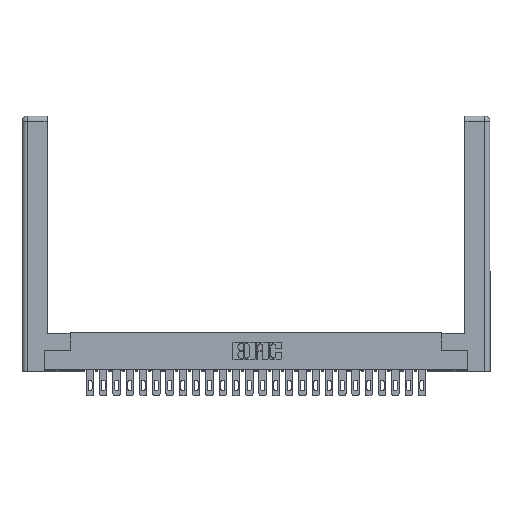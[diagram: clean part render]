
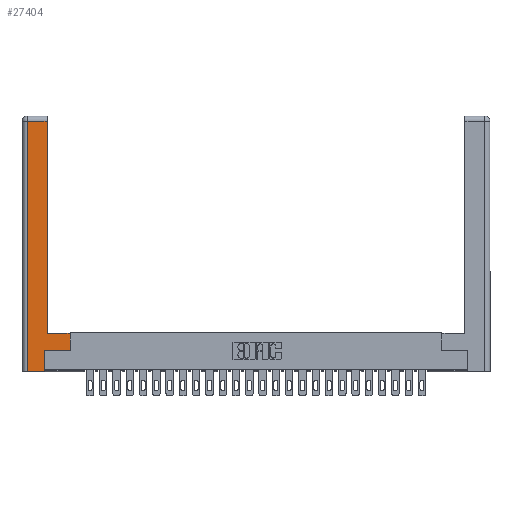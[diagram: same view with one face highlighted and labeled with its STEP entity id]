
A CAD part, top view. The second image highlights one B-rep face of the part: STEP entity #27404.
In plain terms, the highlighted planar face has unit normal (0, 0, 1).
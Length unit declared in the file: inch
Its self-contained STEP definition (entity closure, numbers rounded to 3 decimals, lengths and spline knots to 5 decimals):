
#1443 = ORIENTED_EDGE ( 'NONE', *, *, #8152, .T. ) ;
#1569 = VECTOR ( 'NONE', #4628, 39.37008 ) ;
#1930 = CARTESIAN_POINT ( 'NONE',  ( 0.565, 0.245, 0. ) ) ;
#2510 = VERTEX_POINT ( 'NONE', #10529 ) ;
#3522 = EDGE_CURVE ( 'NONE', #22844, #14500, #9062, .T. ) ;
#3956 = VERTEX_POINT ( 'NONE', #15222 ) ;
#4116 = CARTESIAN_POINT ( 'NONE',  ( 0.265, 0.245, 0. ) ) ;
#4407 = ORIENTED_EDGE ( 'NONE', *, *, #3522, .T. ) ;
#4551 = DIRECTION ( 'NONE',  ( -1., 0., 0. ) ) ;
#4628 = DIRECTION ( 'NONE',  ( -1., 0., 0. ) ) ;
#5605 = EDGE_CURVE ( 'NONE', #5636, #3956, #26532, .T. ) ;
#5636 = VERTEX_POINT ( 'NONE', #1930 ) ;
#5921 = DIRECTION ( 'NONE',  ( 0., -1., 0. ) ) ;
#6219 = DIRECTION ( 'NONE',  ( -1., 0., 0. ) ) ;
#6247 = ORIENTED_EDGE ( 'NONE', *, *, #16109, .T. ) ;
#6635 = CARTESIAN_POINT ( 'NONE',  ( 0.265, 0., 0. ) ) ;
#6903 = AXIS2_PLACEMENT_3D ( 'NONE', #17672, #26797, #4551 ) ;
#7420 = LINE ( 'NONE', #27299, #1569 ) ;
#7659 = ORIENTED_EDGE ( 'NONE', *, *, #13630, .T. ) ;
#7893 = DIRECTION ( 'NONE',  ( 1., 0., 0. ) ) ;
#8052 = VERTEX_POINT ( 'NONE', #11225 ) ;
#8152 = EDGE_CURVE ( 'NONE', #3956, #22844, #7420, .T. ) ;
#8235 = LINE ( 'NONE', #4116, #26697 ) ;
#8256 = EDGE_LOOP ( 'NONE', ( #4407, #15920, #23456, #6247, #7659, #26648, #13505, #1443 ) ) ;
#8911 = DIRECTION ( 'NONE',  ( 0., 1., 0. ) ) ;
#9062 = LINE ( 'NONE', #11106, #13403 ) ;
#10479 = VECTOR ( 'NONE', #7893, 39.37008 ) ;
#10529 = CARTESIAN_POINT ( 'NONE',  ( 0.0615, 0., 0. ) ) ;
#10731 = PLANE ( 'NONE',  #6903 ) ;
#10889 = VECTOR ( 'NONE', #5921, 39.37008 ) ;
#11106 = CARTESIAN_POINT ( 'NONE',  ( 0.295, 3., 0. ) ) ;
#11225 = CARTESIAN_POINT ( 'NONE',  ( 0.0615, 2.94, 0. ) ) ;
#12247 = CARTESIAN_POINT ( 'NONE',  ( 0.295, 0.45, 0. ) ) ;
#12277 = CARTESIAN_POINT ( 'NONE',  ( 0.565, 0.245, 0. ) ) ;
#12647 = CARTESIAN_POINT ( 'NONE',  ( 0.0615, 0., 0. ) ) ;
#12722 = LINE ( 'NONE', #12277, #10479 ) ;
#13403 = VECTOR ( 'NONE', #8911, 39.37008 ) ;
#13505 = ORIENTED_EDGE ( 'NONE', *, *, #5605, .T. ) ;
#13630 = EDGE_CURVE ( 'NONE', #23438, #15552, #8235, .T. ) ;
#14363 = CARTESIAN_POINT ( 'NONE',  ( 0.265, 0.245, 0. ) ) ;
#14500 = VERTEX_POINT ( 'NONE', #28344 ) ;
#15222 = CARTESIAN_POINT ( 'NONE',  ( 0.565, 0.45, 0. ) ) ;
#15308 = FACE_OUTER_BOUND ( 'NONE', #8256, .T. ) ;
#15552 = VERTEX_POINT ( 'NONE', #14363 ) ;
#15601 = DIRECTION ( 'NONE',  ( 1., 0., 0. ) ) ;
#15920 = ORIENTED_EDGE ( 'NONE', *, *, #17751, .T. ) ;
#15979 = VECTOR ( 'NONE', #6219, 39.37008 ) ;
#16109 = EDGE_CURVE ( 'NONE', #2510, #23438, #20025, .T. ) ;
#16445 = CARTESIAN_POINT ( 'NONE',  ( 0.265, 0., 0. ) ) ;
#17672 = CARTESIAN_POINT ( 'NONE',  ( 0., 0., 0. ) ) ;
#17751 = EDGE_CURVE ( 'NONE', #14500, #8052, #28140, .T. ) ;
#20025 = LINE ( 'NONE', #6635, #23934 ) ;
#20279 = EDGE_CURVE ( 'NONE', #8052, #2510, #26665, .T. ) ;
#21168 = EDGE_CURVE ( 'NONE', #15552, #5636, #12722, .T. ) ;
#22095 = DIRECTION ( 'NONE',  ( 0., 1., 0. ) ) ;
#22550 = CARTESIAN_POINT ( 'NONE',  ( 0.565, 0.45, 0. ) ) ;
#22844 = VERTEX_POINT ( 'NONE', #12247 ) ;
#23438 = VERTEX_POINT ( 'NONE', #16445 ) ;
#23456 = ORIENTED_EDGE ( 'NONE', *, *, #20279, .T. ) ;
#23934 = VECTOR ( 'NONE', #15601, 39.37008 ) ;
#24014 = CARTESIAN_POINT ( 'NONE',  ( 0.0615, 2.94, 0. ) ) ;
#24887 = VECTOR ( 'NONE', #26675, 39.37008 ) ;
#26532 = LINE ( 'NONE', #22550, #24887 ) ;
#26648 = ORIENTED_EDGE ( 'NONE', *, *, #21168, .T. ) ;
#26665 = LINE ( 'NONE', #12647, #10889 ) ;
#26675 = DIRECTION ( 'NONE',  ( 0., 1., 0. ) ) ;
#26697 = VECTOR ( 'NONE', #22095, 39.37008 ) ;
#26797 = DIRECTION ( 'NONE',  ( 0., 0., -1. ) ) ;
#27299 = CARTESIAN_POINT ( 'NONE',  ( 0.295, 0.45, 0. ) ) ;
#27404 = ADVANCED_FACE ( 'NONE', ( #15308 ), #10731, .F. ) ;
#28140 = LINE ( 'NONE', #24014, #15979 ) ;
#28344 = CARTESIAN_POINT ( 'NONE',  ( 0.295, 2.94, 0. ) ) ;
